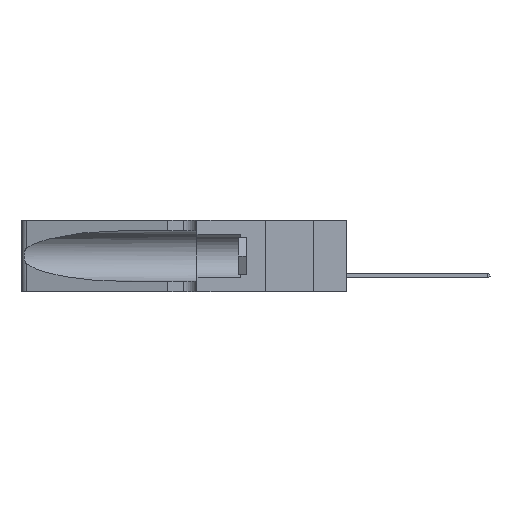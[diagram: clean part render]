
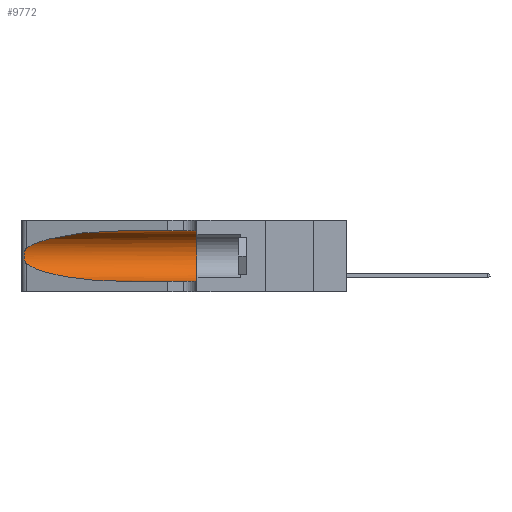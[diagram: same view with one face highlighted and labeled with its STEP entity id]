
A CAD part, left-side view. The second image highlights one B-rep face of the part: STEP entity #9772.
In plain terms, the highlighted cylindrical face has radius 3.308 mm (diameter 6.617 mm), a partial arc.
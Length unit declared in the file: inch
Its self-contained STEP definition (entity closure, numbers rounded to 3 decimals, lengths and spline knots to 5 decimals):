
#196 = CARTESIAN_POINT ( 'NONE',  ( 0.1305, 0.35, 0.05475 ) ) ;
#413 = CARTESIAN_POINT ( 'NONE',  ( 0.25854, 1.2359, 0.20912 ) ) ;
#909 = CARTESIAN_POINT ( 'NONE',  ( 0.18966, 0.96281, 0.05475 ) ) ;
#993 = CARTESIAN_POINT ( 'NONE',  ( 0.25639, 1.23186, 0.15144 ) ) ;
#1089 = CARTESIAN_POINT ( 'NONE',  ( 0.18966, 0.96281, 0.31525 ) ) ;
#1124 = CARTESIAN_POINT ( 'NONE',  ( 0.25487, 1.22718, 0.14631 ) ) ;
#1129 = CARTESIAN_POINT ( 'NONE',  ( 0.1305, 0.35, 0.31525 ) ) ;
#1130 = CARTESIAN_POINT ( 'NONE',  ( 0.1305, 1.61858, 0.185 ) ) ;
#1385 = VERTEX_POINT ( 'NONE', #196 ) ;
#2313 = VERTEX_POINT ( 'NONE', #1129 ) ;
#2483 = CARTESIAN_POINT ( 'NONE',  ( 0.25555, 1.22994, 0.2215 ) ) ;
#2557 = LINE ( 'NONE', #16926, #12305 ) ;
#3377 = DIRECTION ( 'NONE',  ( 0., 0., 1. ) ) ;
#3966 = CARTESIAN_POINT ( 'NONE',  ( 0.1305, 0.72297, 0.31525 ) ) ;
#4102 = AXIS2_PLACEMENT_3D ( 'NONE', #16999, #15050, #3377 ) ;
#4449 = EDGE_CURVE ( 'NONE', #6177, #20773, #6069, .T. ) ;
#4908 = EDGE_CURVE ( 'NONE', #2313, #1385, #11631, .T. ) ;
#5038 = ORIENTED_EDGE ( 'NONE', *, *, #4908, .F. ) ;
#5274 = CARTESIAN_POINT ( 'NONE',  ( 0.25555, 1.22993, 0.14849 ) ) ;
#5312 = ORIENTED_EDGE ( 'NONE', *, *, #9806, .T. ) ;
#6069 =( BOUNDED_CURVE ( )  B_SPLINE_CURVE ( 3, ( #3966, #1089, #15987, #6694 ),
 .UNSPECIFIED., .F., .T. ) 
 B_SPLINE_CURVE_WITH_KNOTS ( ( 4, 4 ),
 ( 1.5708, 2.84003 ),
 .UNSPECIFIED. ) 
 CURVE ( )  GEOMETRIC_REPRESENTATION_ITEM ( )  RATIONAL_B_SPLINE_CURVE ( ( 1., 0.87, 0.87, 1. ) ) 
 REPRESENTATION_ITEM ( '' )  );
#6169 = ORIENTED_EDGE ( 'NONE', *, *, #14757, .T. ) ;
#6177 = VERTEX_POINT ( 'NONE', #12636 ) ;
#6334 = CARTESIAN_POINT ( 'NONE',  ( 0.26075, 1.23896, 0.19203 ) ) ;
#6563 = ORIENTED_EDGE ( 'NONE', *, *, #6662, .T. ) ;
#6662 = EDGE_CURVE ( 'NONE', #25036, #7194, #20421, .T. ) ;
#6694 = CARTESIAN_POINT ( 'NONE',  ( 0.25487, 1.22718, 0.22369 ) ) ;
#7042 = DIRECTION ( 'NONE',  ( 0., -1., 0. ) ) ;
#7194 = VERTEX_POINT ( 'NONE', #10342 ) ;
#7624 = ORIENTED_EDGE ( 'NONE', *, *, #4449, .T. ) ;
#8293 = CARTESIAN_POINT ( 'NONE',  ( 0.26017, 1.23833, 0.17102 ) ) ;
#8743 = CYLINDRICAL_SURFACE ( 'NONE', #23572, 0.13025 ) ;
#8874 = VECTOR ( 'NONE', #18132, 39.37008 ) ;
#9772 = ADVANCED_FACE ( 'NONE', ( #19118 ), #8743, .F. ) ;
#9806 = EDGE_CURVE ( 'NONE', #20773, #25036, #13242, .T. ) ;
#10188 = CARTESIAN_POINT ( 'NONE',  ( 0.25487, 1.22718, 0.22369 ) ) ;
#10342 = CARTESIAN_POINT ( 'NONE',  ( 0.1305, 0.72297, 0.05475 ) ) ;
#10658 = CARTESIAN_POINT ( 'NONE',  ( 0.25487, 1.22718, 0.14631 ) ) ;
#11631 = CIRCLE ( 'NONE', #4102, 0.13025 ) ;
#12105 = CARTESIAN_POINT ( 'NONE',  ( 0.25787, 1.23484, 0.2124 ) ) ;
#12305 = VECTOR ( 'NONE', #17006, 39.37008 ) ;
#12636 = CARTESIAN_POINT ( 'NONE',  ( 0.1305, 0.72297, 0.31525 ) ) ;
#12673 = CARTESIAN_POINT ( 'NONE',  ( 0.1305, 1.61858, 0.31525 ) ) ;
#13242 = B_SPLINE_CURVE_WITH_KNOTS ( 'NONE', 3,
 ( #10188, #2483, #17990, #12105, #413, #14114, #6334, #18072, #8293, #23529, #22153, #993, #5274, #19860 ),
 .UNSPECIFIED., .F., .F.,
 ( 4, 2, 2, 2, 2, 2, 4 ),
 ( 0., 0.00027, 0.00053, 0.00107, 0.0016, 0.00187, 0.00214 ),
 .UNSPECIFIED. ) ;
#14114 = CARTESIAN_POINT ( 'NONE',  ( 0.26018, 1.23835, 0.19895 ) ) ;
#14370 = ORIENTED_EDGE ( 'NONE', *, *, #20582, .F. ) ;
#14757 = EDGE_CURVE ( 'NONE', #7194, #1385, #2557, .T. ) ;
#15050 = DIRECTION ( 'NONE',  ( 0., 1., 0. ) ) ;
#15987 = CARTESIAN_POINT ( 'NONE',  ( 0.2373, 1.15595, 0.28018 ) ) ;
#16292 = CARTESIAN_POINT ( 'NONE',  ( 0.1305, 0.72297, 0.05475 ) ) ;
#16926 = CARTESIAN_POINT ( 'NONE',  ( 0.1305, 1.61858, 0.05475 ) ) ;
#16999 = CARTESIAN_POINT ( 'NONE',  ( 0.1305, 0.35, 0.185 ) ) ;
#17006 = DIRECTION ( 'NONE',  ( 0., -1., 0. ) ) ;
#17236 = DIRECTION ( 'NONE',  ( 0., 0., -1. ) ) ;
#17990 = CARTESIAN_POINT ( 'NONE',  ( 0.25639, 1.23184, 0.21858 ) ) ;
#18072 = CARTESIAN_POINT ( 'NONE',  ( 0.26075, 1.23896, 0.178 ) ) ;
#18132 = DIRECTION ( 'NONE',  ( 0., -1., 0. ) ) ;
#18479 = CARTESIAN_POINT ( 'NONE',  ( 0.2373, 1.15595, 0.08982 ) ) ;
#19056 = EDGE_LOOP ( 'NONE', ( #7624, #5312, #6563, #6169, #5038, #14370 ) ) ;
#19118 = FACE_OUTER_BOUND ( 'NONE', #19056, .T. ) ;
#19860 = CARTESIAN_POINT ( 'NONE',  ( 0.25487, 1.22718, 0.14631 ) ) ;
#20421 =( BOUNDED_CURVE ( )  B_SPLINE_CURVE ( 3, ( #10658, #18479, #909, #16292 ),
 .UNSPECIFIED., .F., .T. ) 
 B_SPLINE_CURVE_WITH_KNOTS ( ( 4, 4 ),
 ( 3.44316, 4.71239 ),
 .UNSPECIFIED. ) 
 CURVE ( )  GEOMETRIC_REPRESENTATION_ITEM ( )  RATIONAL_B_SPLINE_CURVE ( ( 1., 0.87, 0.87, 1. ) ) 
 REPRESENTATION_ITEM ( '' )  );
#20500 = CARTESIAN_POINT ( 'NONE',  ( 0.25487, 1.22718, 0.22369 ) ) ;
#20582 = EDGE_CURVE ( 'NONE', #6177, #2313, #21926, .T. ) ;
#20773 = VERTEX_POINT ( 'NONE', #20500 ) ;
#21926 = LINE ( 'NONE', #12673, #8874 ) ;
#22153 = CARTESIAN_POINT ( 'NONE',  ( 0.25789, 1.23486, 0.15765 ) ) ;
#23529 = CARTESIAN_POINT ( 'NONE',  ( 0.25856, 1.23593, 0.16098 ) ) ;
#23572 = AXIS2_PLACEMENT_3D ( 'NONE', #1130, #7042, #17236 ) ;
#25036 = VERTEX_POINT ( 'NONE', #1124 ) ;
